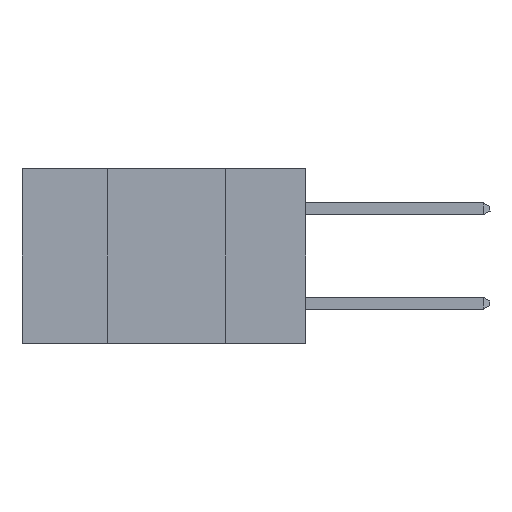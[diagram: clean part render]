
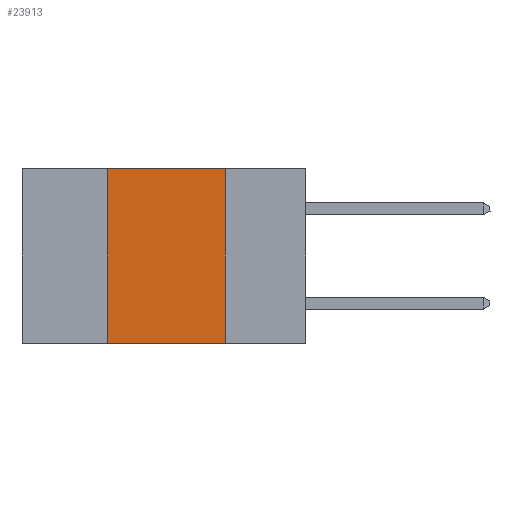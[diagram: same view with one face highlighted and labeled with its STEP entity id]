
A CAD part, left-side view. The second image highlights one B-rep face of the part: STEP entity #23913.
In plain terms, the highlighted planar face has unit normal (-1, 0, 0).
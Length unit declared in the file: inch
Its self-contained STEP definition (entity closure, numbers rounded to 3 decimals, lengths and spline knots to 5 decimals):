
#134 = DIRECTION ( 'NONE',  ( 0., -1., 0. ) ) ;
#385 = VERTEX_POINT ( 'NONE', #26172 ) ;
#2022 = VECTOR ( 'NONE', #6447, 39.37008 ) ;
#2863 = VECTOR ( 'NONE', #21628, 39.37008 ) ;
#3126 = VECTOR ( 'NONE', #134, 39.37008 ) ;
#4002 = LINE ( 'NONE', #29340, #2863 ) ;
#4152 = CARTESIAN_POINT ( 'NONE',  ( 0., 0.42, 0. ) ) ;
#5490 = VECTOR ( 'NONE', #22763, 39.37008 ) ;
#6447 = DIRECTION ( 'NONE',  ( 0., -1., 0. ) ) ;
#7720 = CARTESIAN_POINT ( 'NONE',  ( 0., 0.6, 0. ) ) ;
#8066 = EDGE_CURVE ( 'NONE', #21796, #29404, #17905, .T. ) ;
#9106 = AXIS2_PLACEMENT_3D ( 'NONE', #11715, #28622, #31049 ) ;
#9998 = LINE ( 'NONE', #30317, #2022 ) ;
#10044 = LINE ( 'NONE', #10735, #5490 ) ;
#10735 = CARTESIAN_POINT ( 'NONE',  ( 0., 0.17, 0. ) ) ;
#11611 = PLANE ( 'NONE',  #9106 ) ;
#11715 = CARTESIAN_POINT ( 'NONE',  ( 0., 0.6, 0. ) ) ;
#16974 = EDGE_CURVE ( 'NONE', #385, #21796, #4002, .T. ) ;
#17866 = EDGE_LOOP ( 'NONE', ( #23466, #23334, #24447, #31072 ) ) ;
#17905 = LINE ( 'NONE', #7720, #3126 ) ;
#21011 = VERTEX_POINT ( 'NONE', #29398 ) ;
#21628 = DIRECTION ( 'NONE',  ( 0., 0., 1. ) ) ;
#21796 = VERTEX_POINT ( 'NONE', #4152 ) ;
#22763 = DIRECTION ( 'NONE',  ( 0., 0., -1. ) ) ;
#23334 = ORIENTED_EDGE ( 'NONE', *, *, #8066, .F. ) ;
#23466 = ORIENTED_EDGE ( 'NONE', *, *, #29369, .F. ) ;
#23679 = EDGE_CURVE ( 'NONE', #385, #21011, #9998, .T. ) ;
#23913 = ADVANCED_FACE ( 'NONE', ( #29265 ), #11611, .F. ) ;
#24447 = ORIENTED_EDGE ( 'NONE', *, *, #16974, .F. ) ;
#26172 = CARTESIAN_POINT ( 'NONE',  ( 0., 0.42, -0.37 ) ) ;
#28622 = DIRECTION ( 'NONE',  ( 1., 0., 0. ) ) ;
#29265 = FACE_OUTER_BOUND ( 'NONE', #17866, .T. ) ;
#29340 = CARTESIAN_POINT ( 'NONE',  ( 0., 0.42, 0. ) ) ;
#29369 = EDGE_CURVE ( 'NONE', #29404, #21011, #10044, .T. ) ;
#29398 = CARTESIAN_POINT ( 'NONE',  ( 0., 0.17, -0.37 ) ) ;
#29404 = VERTEX_POINT ( 'NONE', #29955 ) ;
#29955 = CARTESIAN_POINT ( 'NONE',  ( 0., 0.17, 0. ) ) ;
#30317 = CARTESIAN_POINT ( 'NONE',  ( 0., 0.6, -0.37 ) ) ;
#31049 = DIRECTION ( 'NONE',  ( 0., 0., -1. ) ) ;
#31072 = ORIENTED_EDGE ( 'NONE', *, *, #23679, .T. ) ;
